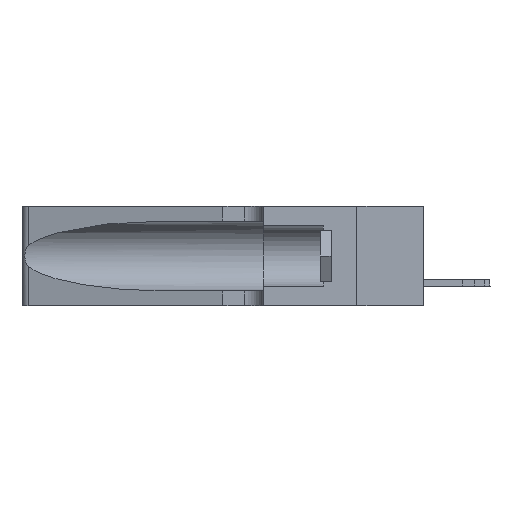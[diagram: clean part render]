
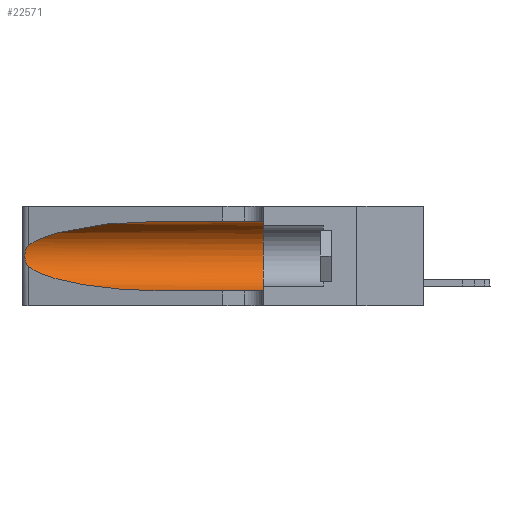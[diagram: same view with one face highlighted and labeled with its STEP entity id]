
A CAD part, left-side view. The second image highlights one B-rep face of the part: STEP entity #22571.
In plain terms, the highlighted cylindrical face has radius 3.308 mm (diameter 6.617 mm), a partial arc.
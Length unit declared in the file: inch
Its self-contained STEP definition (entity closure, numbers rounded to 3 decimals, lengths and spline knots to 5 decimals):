
#45 = CARTESIAN_POINT ( 'NONE',  ( 0.25787, 1.23484, 0.2124 ) ) ;
#2859 = VERTEX_POINT ( 'NONE', #22674 ) ;
#3069 =( BOUNDED_CURVE ( )  B_SPLINE_CURVE ( 3, ( #20341, #20440, #20542, #25081 ),
 .UNSPECIFIED., .F., .F. ) 
 B_SPLINE_CURVE_WITH_KNOTS ( ( 4, 4 ),
 ( 1.5708, 2.84003 ),
 .UNSPECIFIED. ) 
 CURVE ( )  GEOMETRIC_REPRESENTATION_ITEM ( )  RATIONAL_B_SPLINE_CURVE ( ( 1., 0.87, 0.87, 1. ) ) 
 REPRESENTATION_ITEM ( '' )  );
#3147 = CARTESIAN_POINT ( 'NONE',  ( 0.1305, 1.61858, 0.05475 ) ) ;
#4194 = VERTEX_POINT ( 'NONE', #28012 ) ;
#4467 = AXIS2_PLACEMENT_3D ( 'NONE', #19803, #15370, #27019 ) ;
#4606 = CARTESIAN_POINT ( 'NONE',  ( 0.25487, 1.22718, 0.14631 ) ) ;
#4694 = EDGE_CURVE ( 'NONE', #23550, #2859, #15037, .T. ) ;
#8467 = CARTESIAN_POINT ( 'NONE',  ( 0.1305, 1.61858, 0.185 ) ) ;
#8602 = CARTESIAN_POINT ( 'NONE',  ( 0.2373, 1.15595, 0.08982 ) ) ;
#8895 = CARTESIAN_POINT ( 'NONE',  ( 0.18966, 0.96281, 0.05475 ) ) ;
#9346 = CARTESIAN_POINT ( 'NONE',  ( 0.25487, 1.22718, 0.22369 ) ) ;
#9634 = CARTESIAN_POINT ( 'NONE',  ( 0.25854, 1.2359, 0.20912 ) ) ;
#10131 = EDGE_LOOP ( 'NONE', ( #16602, #23435, #11408, #29206, #25044, #10759 ) ) ;
#10296 = VERTEX_POINT ( 'NONE', #25327 ) ;
#10376 = EDGE_CURVE ( 'NONE', #26760, #10296, #19064, .T. ) ;
#10759 = ORIENTED_EDGE ( 'NONE', *, *, #10376, .F. ) ;
#10937 = DIRECTION ( 'NONE',  ( 0., -1., 0. ) ) ;
#11408 = ORIENTED_EDGE ( 'NONE', *, *, #17737, .T. ) ;
#11702 = CARTESIAN_POINT ( 'NONE',  ( 0.25639, 1.23184, 0.21858 ) ) ;
#11938 = CARTESIAN_POINT ( 'NONE',  ( 0.25487, 1.22718, 0.22369 ) ) ;
#11988 = CARTESIAN_POINT ( 'NONE',  ( 0.26017, 1.23833, 0.17102 ) ) ;
#13145 = VECTOR ( 'NONE', #28060, 39.37008 ) ;
#13677 = EDGE_CURVE ( 'NONE', #10296, #2859, #14457, .T. ) ;
#14457 = CIRCLE ( 'NONE', #4467, 0.13025 ) ;
#14517 = EDGE_CURVE ( 'NONE', #26760, #30499, #3069, .T. ) ;
#15037 = LINE ( 'NONE', #3147, #28655 ) ;
#15370 = DIRECTION ( 'NONE',  ( 0., 1., 0. ) ) ;
#15652 = CARTESIAN_POINT ( 'NONE',  ( 0.25487, 1.22718, 0.14631 ) ) ;
#16024 = CARTESIAN_POINT ( 'NONE',  ( 0.1305, 0.72297, 0.31525 ) ) ;
#16471 = CARTESIAN_POINT ( 'NONE',  ( 0.25555, 1.22993, 0.14849 ) ) ;
#16602 = ORIENTED_EDGE ( 'NONE', *, *, #14517, .T. ) ;
#17301 = CARTESIAN_POINT ( 'NONE',  ( 0.26075, 1.23896, 0.19203 ) ) ;
#17470 =( BOUNDED_CURVE ( )  B_SPLINE_CURVE ( 3, ( #15652, #8602, #8895, #20682 ),
 .UNSPECIFIED., .F., .T. ) 
 B_SPLINE_CURVE_WITH_KNOTS ( ( 4, 4 ),
 ( 3.44316, 4.71239 ),
 .UNSPECIFIED. ) 
 CURVE ( )  GEOMETRIC_REPRESENTATION_ITEM ( )  RATIONAL_B_SPLINE_CURVE ( ( 1., 0.87, 0.87, 1. ) ) 
 REPRESENTATION_ITEM ( '' )  );
#17737 = EDGE_CURVE ( 'NONE', #4194, #23550, #17470, .T. ) ;
#18844 = CARTESIAN_POINT ( 'NONE',  ( 0.25555, 1.22994, 0.2215 ) ) ;
#19064 = LINE ( 'NONE', #25575, #13145 ) ;
#19803 = CARTESIAN_POINT ( 'NONE',  ( 0.1305, 0.35, 0.185 ) ) ;
#19895 = B_SPLINE_CURVE_WITH_KNOTS ( 'NONE', 3,
 ( #9346, #18844, #11702, #45, #9634, #23536, #17301, #28231, #11988, #23838, #30630, #26244, #16471, #4606 ),
 .UNSPECIFIED., .F., .F.,
 ( 4, 2, 2, 2, 2, 2, 4 ),
 ( 0., 0.00027, 0.00053, 0.00107, 0.0016, 0.00187, 0.00214 ),
 .UNSPECIFIED. ) ;
#20341 = CARTESIAN_POINT ( 'NONE',  ( 0.1305, 0.72297, 0.31525 ) ) ;
#20440 = CARTESIAN_POINT ( 'NONE',  ( 0.18966, 0.96281, 0.31525 ) ) ;
#20542 = CARTESIAN_POINT ( 'NONE',  ( 0.2373, 1.15595, 0.28018 ) ) ;
#20682 = CARTESIAN_POINT ( 'NONE',  ( 0.1305, 0.72297, 0.05475 ) ) ;
#21386 = EDGE_CURVE ( 'NONE', #30499, #4194, #19895, .T. ) ;
#22033 = AXIS2_PLACEMENT_3D ( 'NONE', #8467, #10937, #27256 ) ;
#22571 = ADVANCED_FACE ( 'NONE', ( #25512 ), #24402, .F. ) ;
#22674 = CARTESIAN_POINT ( 'NONE',  ( 0.1305, 0.35, 0.05475 ) ) ;
#23435 = ORIENTED_EDGE ( 'NONE', *, *, #21386, .T. ) ;
#23536 = CARTESIAN_POINT ( 'NONE',  ( 0.26018, 1.23835, 0.19895 ) ) ;
#23550 = VERTEX_POINT ( 'NONE', #24531 ) ;
#23838 = CARTESIAN_POINT ( 'NONE',  ( 0.25856, 1.23593, 0.16098 ) ) ;
#24402 = CYLINDRICAL_SURFACE ( 'NONE', #22033, 0.13025 ) ;
#24409 = DIRECTION ( 'NONE',  ( 0., -1., 0. ) ) ;
#24531 = CARTESIAN_POINT ( 'NONE',  ( 0.1305, 0.72297, 0.05475 ) ) ;
#25044 = ORIENTED_EDGE ( 'NONE', *, *, #13677, .F. ) ;
#25081 = CARTESIAN_POINT ( 'NONE',  ( 0.25487, 1.22718, 0.22369 ) ) ;
#25327 = CARTESIAN_POINT ( 'NONE',  ( 0.1305, 0.35, 0.31525 ) ) ;
#25512 = FACE_OUTER_BOUND ( 'NONE', #10131, .T. ) ;
#25575 = CARTESIAN_POINT ( 'NONE',  ( 0.1305, 1.61858, 0.31525 ) ) ;
#26244 = CARTESIAN_POINT ( 'NONE',  ( 0.25639, 1.23186, 0.15144 ) ) ;
#26760 = VERTEX_POINT ( 'NONE', #16024 ) ;
#27019 = DIRECTION ( 'NONE',  ( 0., 0., 1. ) ) ;
#27256 = DIRECTION ( 'NONE',  ( 0., 0., -1. ) ) ;
#28012 = CARTESIAN_POINT ( 'NONE',  ( 0.25487, 1.22718, 0.14631 ) ) ;
#28060 = DIRECTION ( 'NONE',  ( 0., -1., 0. ) ) ;
#28231 = CARTESIAN_POINT ( 'NONE',  ( 0.26075, 1.23896, 0.178 ) ) ;
#28655 = VECTOR ( 'NONE', #24409, 39.37008 ) ;
#29206 = ORIENTED_EDGE ( 'NONE', *, *, #4694, .T. ) ;
#30499 = VERTEX_POINT ( 'NONE', #11938 ) ;
#30630 = CARTESIAN_POINT ( 'NONE',  ( 0.25789, 1.23486, 0.15765 ) ) ;
